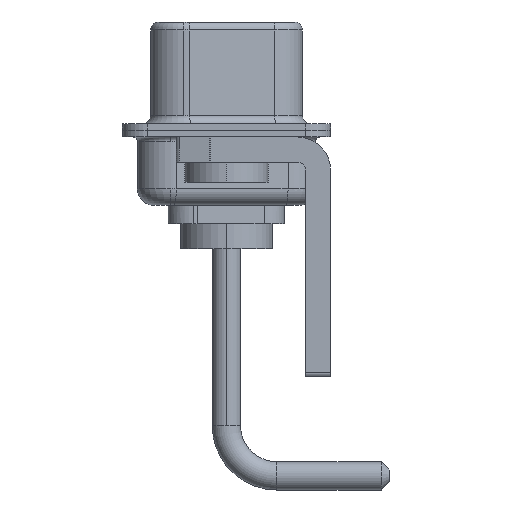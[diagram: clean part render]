
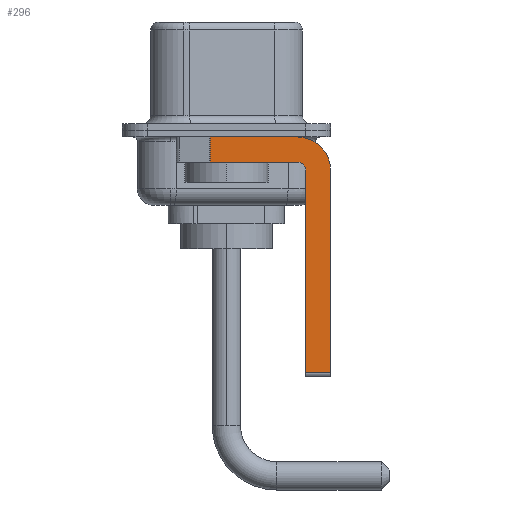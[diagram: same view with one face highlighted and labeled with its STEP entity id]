
A CAD part, left-side view. The second image highlights one B-rep face of the part: STEP entity #296.
In plain terms, the highlighted planar face has unit normal (-1, 0, 0).
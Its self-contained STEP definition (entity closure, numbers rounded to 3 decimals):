
#296 = ADVANCED_FACE ( 'NONE', ( #7727 ), #15170, .F. ) ;
#341 = ORIENTED_EDGE ( 'NONE', *, *, #5508, .F. ) ;
#792 = ORIENTED_EDGE ( 'NONE', *, *, #14447, .F. ) ;
#1104 = VERTEX_POINT ( 'NONE', #1461 ) ;
#1461 = CARTESIAN_POINT ( 'NONE',  ( -2.9, -6.25, -2.4 ) ) ;
#1472 = CARTESIAN_POINT ( 'NONE',  ( -2.9, -4.75, -2.4 ) ) ;
#1740 = LINE ( 'NONE', #5154, #14720 ) ;
#1751 = VECTOR ( 'NONE', #5662, 1000. ) ;
#1960 = CARTESIAN_POINT ( 'NONE',  ( -2.9, -4.25, -2.4 ) ) ;
#1973 = VERTEX_POINT ( 'NONE', #9014 ) ;
#2453 = ORIENTED_EDGE ( 'NONE', *, *, #11788, .T. ) ;
#3051 = DIRECTION ( 'NONE',  ( -1., 0., 0. ) ) ;
#3055 = EDGE_CURVE ( 'NONE', #1104, #13467, #3092, .T. ) ;
#3092 = LINE ( 'NONE', #7828, #9619 ) ;
#4050 = VECTOR ( 'NONE', #11999, 1000. ) ;
#4323 = VERTEX_POINT ( 'NONE', #1472 ) ;
#4669 = DIRECTION ( 'NONE',  ( 0., 0., -1. ) ) ;
#4742 = VERTEX_POINT ( 'NONE', #15268 ) ;
#5154 = CARTESIAN_POINT ( 'NONE',  ( -2.9, -4.25, -1.9 ) ) ;
#5234 = CARTESIAN_POINT ( 'NONE',  ( -2.9, 0.978, -0.4 ) ) ;
#5508 = EDGE_CURVE ( 'NONE', #4323, #8581, #9372, .T. ) ;
#5562 = VERTEX_POINT ( 'NONE', #5234 ) ;
#5599 = EDGE_CURVE ( 'NONE', #14570, #1104, #12626, .T. ) ;
#5662 = DIRECTION ( 'NONE',  ( 0., 0., -1. ) ) ;
#5710 = ORIENTED_EDGE ( 'NONE', *, *, #3055, .F. ) ;
#6643 = AXIS2_PLACEMENT_3D ( 'NONE', #8725, #3051, #7788 ) ;
#6658 = DIRECTION ( 'NONE',  ( 0., 0., -1. ) ) ;
#6785 = CARTESIAN_POINT ( 'NONE',  ( -2.9, -4.25, -2.4 ) ) ;
#7080 = DIRECTION ( 'NONE',  ( 0., -1., 0. ) ) ;
#7290 = EDGE_CURVE ( 'NONE', #5562, #4742, #10333, .T. ) ;
#7727 = FACE_OUTER_BOUND ( 'NONE', #9371, .T. ) ;
#7788 = DIRECTION ( 'NONE',  ( 0., 0., 1. ) ) ;
#7801 = DIRECTION ( 'NONE',  ( 0., 0., -1. ) ) ;
#7828 = CARTESIAN_POINT ( 'NONE',  ( -2.9, -6.25, -2.4 ) ) ;
#7931 = LINE ( 'NONE', #13005, #13254 ) ;
#8051 = CARTESIAN_POINT ( 'NONE',  ( -2.9, -6.25, -14.55 ) ) ;
#8333 = CARTESIAN_POINT ( 'NONE',  ( -2.9, -4.25, -1.9 ) ) ;
#8404 = ORIENTED_EDGE ( 'NONE', *, *, #7290, .T. ) ;
#8499 = CARTESIAN_POINT ( 'NONE',  ( -2.9, -4.25, -0.4 ) ) ;
#8581 = VERTEX_POINT ( 'NONE', #8333 ) ;
#8725 = CARTESIAN_POINT ( 'NONE',  ( -2.9, -4.25, -2.4 ) ) ;
#9014 = CARTESIAN_POINT ( 'NONE',  ( -2.9, -4.75, -14.55 ) ) ;
#9371 = EDGE_LOOP ( 'NONE', ( #11589, #8404, #13290, #341, #792, #2453, #5710, #10892 ) ) ;
#9372 = CIRCLE ( 'NONE', #6643, 0.5 ) ;
#9533 = AXIS2_PLACEMENT_3D ( 'NONE', #6785, #11379, #7801 ) ;
#9619 = VECTOR ( 'NONE', #6658, 1000. ) ;
#10017 = EDGE_CURVE ( 'NONE', #8581, #4742, #1740, .T. ) ;
#10333 = LINE ( 'NONE', #12901, #1751 ) ;
#10892 = ORIENTED_EDGE ( 'NONE', *, *, #5599, .F. ) ;
#11301 = DIRECTION ( 'NONE',  ( 0., 1., 0. ) ) ;
#11379 = DIRECTION ( 'NONE',  ( 1., 0., 0. ) ) ;
#11438 = VECTOR ( 'NONE', #12158, 1000. ) ;
#11589 = ORIENTED_EDGE ( 'NONE', *, *, #11620, .F. ) ;
#11620 = EDGE_CURVE ( 'NONE', #5562, #14570, #7931, .T. ) ;
#11788 = EDGE_CURVE ( 'NONE', #1973, #13467, #12142, .T. ) ;
#11999 = DIRECTION ( 'NONE',  ( 0., -1., 0. ) ) ;
#12142 = LINE ( 'NONE', #13077, #4050 ) ;
#12158 = DIRECTION ( 'NONE',  ( 0., 0., 1. ) ) ;
#12626 = CIRCLE ( 'NONE', #12875, 2. ) ;
#12767 = DIRECTION ( 'NONE',  ( 1., 0., 0. ) ) ;
#12875 = AXIS2_PLACEMENT_3D ( 'NONE', #1960, #12767, #4669 ) ;
#12901 = CARTESIAN_POINT ( 'NONE',  ( -2.9, 0.978, -1.9 ) ) ;
#13005 = CARTESIAN_POINT ( 'NONE',  ( -2.9, 3., -0.4 ) ) ;
#13077 = CARTESIAN_POINT ( 'NONE',  ( -2.9, -4.25, -14.55 ) ) ;
#13178 = CARTESIAN_POINT ( 'NONE',  ( -2.9, -4.75, -14.8 ) ) ;
#13254 = VECTOR ( 'NONE', #7080, 1000. ) ;
#13290 = ORIENTED_EDGE ( 'NONE', *, *, #10017, .F. ) ;
#13467 = VERTEX_POINT ( 'NONE', #8051 ) ;
#14447 = EDGE_CURVE ( 'NONE', #1973, #4323, #14490, .T. ) ;
#14490 = LINE ( 'NONE', #13178, #11438 ) ;
#14570 = VERTEX_POINT ( 'NONE', #8499 ) ;
#14720 = VECTOR ( 'NONE', #11301, 1000. ) ;
#15170 = PLANE ( 'NONE',  #9533 ) ;
#15268 = CARTESIAN_POINT ( 'NONE',  ( -2.9, 0.978, -1.9 ) ) ;
